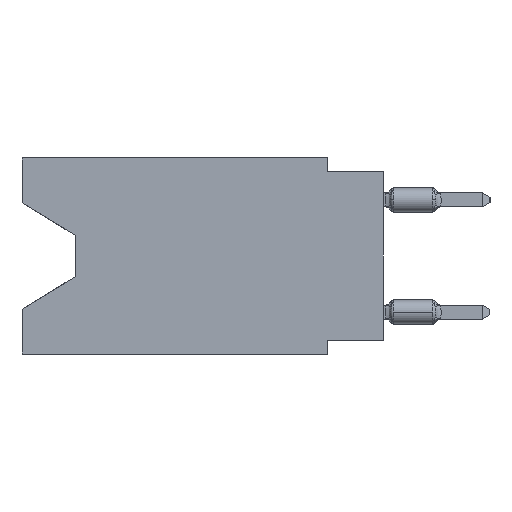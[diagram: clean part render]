
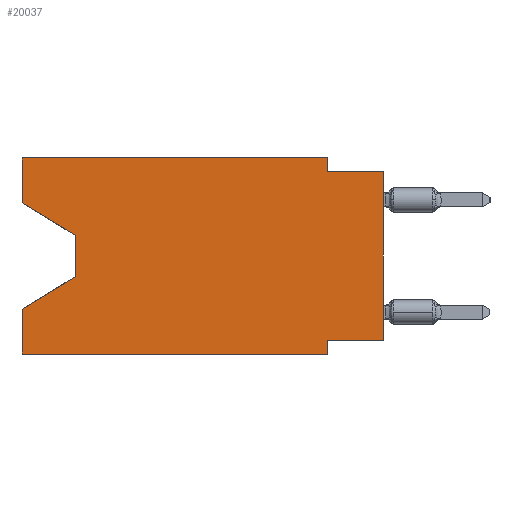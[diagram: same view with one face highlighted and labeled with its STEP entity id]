
A CAD part, left-side view. The second image highlights one B-rep face of the part: STEP entity #20037.
In plain terms, the highlighted planar face has unit normal (-1, 0, 0).
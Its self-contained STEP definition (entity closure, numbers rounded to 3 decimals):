
#447 = LINE ( 'NONE', #21278, #20427 ) ;
#700 = EDGE_CURVE ( 'NONE', #12410, #1218, #10963, .T. ) ;
#960 = DIRECTION ( 'NONE',  ( 0., 0., -1. ) ) ;
#1203 = CARTESIAN_POINT ( 'NONE',  ( 0., 16.383, 0. ) ) ;
#1218 = VERTEX_POINT ( 'NONE', #18883 ) ;
#1309 = CARTESIAN_POINT ( 'NONE',  ( 0., 16.383, -8.89 ) ) ;
#1367 = DIRECTION ( 'NONE',  ( 0., 0., -1. ) ) ;
#1420 = VERTEX_POINT ( 'NONE', #17630 ) ;
#1759 = DIRECTION ( 'NONE',  ( 0., 1., 0. ) ) ;
#2321 = CARTESIAN_POINT ( 'NONE',  ( 0., 0., 0. ) ) ;
#2516 = ORIENTED_EDGE ( 'NONE', *, *, #23168, .F. ) ;
#2561 = DIRECTION ( 'NONE',  ( 0., 0., 1. ) ) ;
#3296 = EDGE_CURVE ( 'NONE', #21739, #19852, #10982, .T. ) ;
#3493 = CARTESIAN_POINT ( 'NONE',  ( 0., 16.383, -2.038 ) ) ;
#3567 = LINE ( 'NONE', #1309, #18614 ) ;
#4136 = EDGE_CURVE ( 'NONE', #13485, #1218, #3567, .T. ) ;
#4431 = VECTOR ( 'NONE', #1367, 1000. ) ;
#4679 = CARTESIAN_POINT ( 'NONE',  ( 0., 16.383, 0. ) ) ;
#4719 = ORIENTED_EDGE ( 'NONE', *, *, #4136, .T. ) ;
#5225 = LINE ( 'NONE', #3493, #22871 ) ;
#5694 = ORIENTED_EDGE ( 'NONE', *, *, #700, .F. ) ;
#5853 = CARTESIAN_POINT ( 'NONE',  ( 0., 13.97, -5.385 ) ) ;
#5953 = LINE ( 'NONE', #9811, #8612 ) ;
#6053 = VECTOR ( 'NONE', #1759, 1000. ) ;
#6672 = DIRECTION ( 'NONE',  ( 0., 0., 1. ) ) ;
#6709 = FACE_OUTER_BOUND ( 'NONE', #13470, .T. ) ;
#6730 = CARTESIAN_POINT ( 'NONE',  ( 0., 2.54, -8.89 ) ) ;
#6994 = CARTESIAN_POINT ( 'NONE',  ( 0., 13.97, -3.505 ) ) ;
#7089 = DIRECTION ( 'NONE',  ( 1., 0., 0. ) ) ;
#7112 = DIRECTION ( 'NONE',  ( 0., -0.855, -0.519 ) ) ;
#7118 = CARTESIAN_POINT ( 'NONE',  ( 0., 13.97, -5.385 ) ) ;
#7246 = CARTESIAN_POINT ( 'NONE',  ( 0., 16.383, -8.89 ) ) ;
#7443 = CARTESIAN_POINT ( 'NONE',  ( 0., 13.97, -3.505 ) ) ;
#8283 = VERTEX_POINT ( 'NONE', #22755 ) ;
#8612 = VECTOR ( 'NONE', #19404, 1000. ) ;
#9049 = ORIENTED_EDGE ( 'NONE', *, *, #13413, .F. ) ;
#9379 = EDGE_CURVE ( 'NONE', #19852, #23746, #16087, .T. ) ;
#9811 = CARTESIAN_POINT ( 'NONE',  ( 0., 16.383, 0. ) ) ;
#10463 = VECTOR ( 'NONE', #6672, 1000. ) ;
#10484 = VECTOR ( 'NONE', #18682, 1000. ) ;
#10569 = PLANE ( 'NONE',  #18518 ) ;
#10891 = CARTESIAN_POINT ( 'NONE',  ( 0., 0., -8.255 ) ) ;
#10963 = LINE ( 'NONE', #6730, #10484 ) ;
#10982 = LINE ( 'NONE', #6994, #17379 ) ;
#11115 = LINE ( 'NONE', #24443, #4431 ) ;
#11217 = EDGE_CURVE ( 'NONE', #8283, #1420, #11943, .T. ) ;
#11806 = ORIENTED_EDGE ( 'NONE', *, *, #15147, .F. ) ;
#11943 = LINE ( 'NONE', #2321, #21481 ) ;
#12410 = VERTEX_POINT ( 'NONE', #21059 ) ;
#12553 = DIRECTION ( 'NONE',  ( 0., -1., 0. ) ) ;
#12976 = DIRECTION ( 'NONE',  ( 0., 0., -1. ) ) ;
#13262 = ORIENTED_EDGE ( 'NONE', *, *, #14047, .F. ) ;
#13413 = EDGE_CURVE ( 'NONE', #24082, #24144, #11115, .T. ) ;
#13470 = EDGE_LOOP ( 'NONE', ( #21589, #22709, #19024, #11806, #4719, #5694, #13262, #16548, #2516, #9049, #23842, #17163 ) ) ;
#13485 = VERTEX_POINT ( 'NONE', #7246 ) ;
#14047 = EDGE_CURVE ( 'NONE', #8283, #12410, #24599, .T. ) ;
#14049 = DIRECTION ( 'NONE',  ( 0., 0., 1. ) ) ;
#14505 = CARTESIAN_POINT ( 'NONE',  ( 0., 0., -0.635 ) ) ;
#14720 = DIRECTION ( 'NONE',  ( 0., 0.855, -0.519 ) ) ;
#15147 = EDGE_CURVE ( 'NONE', #13485, #23746, #20244, .T. ) ;
#16087 = LINE ( 'NONE', #7118, #21080 ) ;
#16548 = ORIENTED_EDGE ( 'NONE', *, *, #11217, .T. ) ;
#16854 = LINE ( 'NONE', #14505, #16981 ) ;
#16981 = VECTOR ( 'NONE', #22590, 1000. ) ;
#17134 = CARTESIAN_POINT ( 'NONE',  ( 0., 16.383, 0. ) ) ;
#17163 = ORIENTED_EDGE ( 'NONE', *, *, #24346, .F. ) ;
#17352 = EDGE_CURVE ( 'NONE', #18573, #21739, #5225, .T. ) ;
#17379 = VECTOR ( 'NONE', #12976, 1000. ) ;
#17630 = CARTESIAN_POINT ( 'NONE',  ( 0., 0., -0.635 ) ) ;
#17867 = VERTEX_POINT ( 'NONE', #17134 ) ;
#18518 = AXIS2_PLACEMENT_3D ( 'NONE', #1203, #7089, #960 ) ;
#18573 = VERTEX_POINT ( 'NONE', #18798 ) ;
#18614 = VECTOR ( 'NONE', #12553, 1000. ) ;
#18682 = DIRECTION ( 'NONE',  ( 0., 0., -1. ) ) ;
#18798 = CARTESIAN_POINT ( 'NONE',  ( 0., 16.383, -2.038 ) ) ;
#18812 = CARTESIAN_POINT ( 'NONE',  ( 0., 16.383, -6.852 ) ) ;
#18883 = CARTESIAN_POINT ( 'NONE',  ( 0., 2.54, -8.89 ) ) ;
#19024 = ORIENTED_EDGE ( 'NONE', *, *, #9379, .T. ) ;
#19404 = DIRECTION ( 'NONE',  ( 0., -1., 0. ) ) ;
#19852 = VERTEX_POINT ( 'NONE', #5853 ) ;
#20037 = ADVANCED_FACE ( 'NONE', ( #6709 ), #10569, .F. ) ;
#20244 = LINE ( 'NONE', #4679, #10463 ) ;
#20427 = VECTOR ( 'NONE', #14049, 1000. ) ;
#21059 = CARTESIAN_POINT ( 'NONE',  ( 0., 2.54, -8.255 ) ) ;
#21080 = VECTOR ( 'NONE', #14720, 1000. ) ;
#21278 = CARTESIAN_POINT ( 'NONE',  ( 0., 16.383, 0. ) ) ;
#21481 = VECTOR ( 'NONE', #2561, 1000. ) ;
#21589 = ORIENTED_EDGE ( 'NONE', *, *, #17352, .T. ) ;
#21739 = VERTEX_POINT ( 'NONE', #7443 ) ;
#22290 = CARTESIAN_POINT ( 'NONE',  ( 0., 2.54, 0. ) ) ;
#22590 = DIRECTION ( 'NONE',  ( 0., -1., 0. ) ) ;
#22653 = CARTESIAN_POINT ( 'NONE',  ( 0., 2.54, -0.635 ) ) ;
#22709 = ORIENTED_EDGE ( 'NONE', *, *, #3296, .T. ) ;
#22755 = CARTESIAN_POINT ( 'NONE',  ( 0., 0., -8.255 ) ) ;
#22871 = VECTOR ( 'NONE', #7112, 1000. ) ;
#23085 = EDGE_CURVE ( 'NONE', #17867, #24082, #5953, .T. ) ;
#23168 = EDGE_CURVE ( 'NONE', #24144, #1420, #16854, .T. ) ;
#23746 = VERTEX_POINT ( 'NONE', #18812 ) ;
#23842 = ORIENTED_EDGE ( 'NONE', *, *, #23085, .F. ) ;
#24082 = VERTEX_POINT ( 'NONE', #22290 ) ;
#24144 = VERTEX_POINT ( 'NONE', #22653 ) ;
#24346 = EDGE_CURVE ( 'NONE', #18573, #17867, #447, .T. ) ;
#24443 = CARTESIAN_POINT ( 'NONE',  ( 0., 2.54, 0. ) ) ;
#24599 = LINE ( 'NONE', #10891, #6053 ) ;
